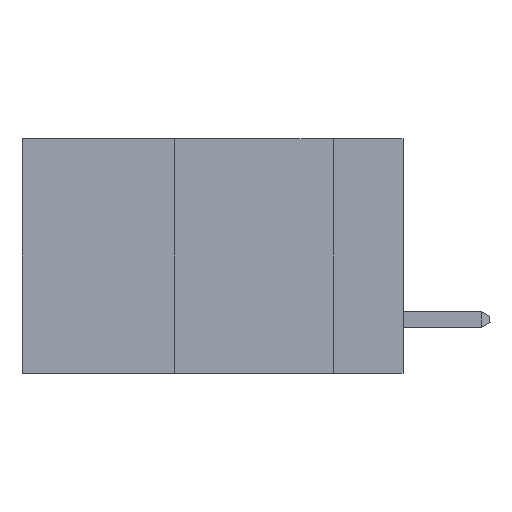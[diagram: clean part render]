
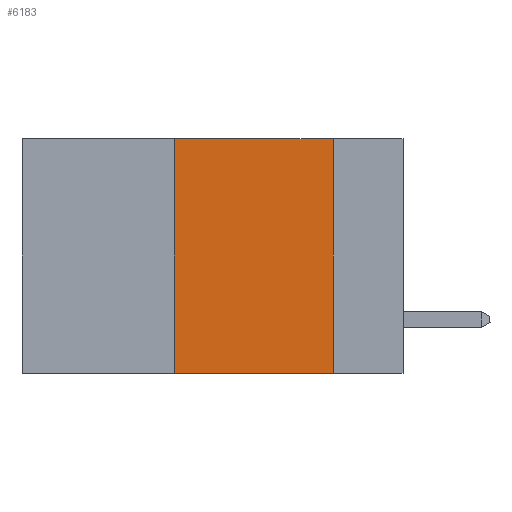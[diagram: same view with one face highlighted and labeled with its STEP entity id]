
A CAD part, left-side view. The second image highlights one B-rep face of the part: STEP entity #6183.
In plain terms, the highlighted planar face has unit normal (-1, 0, 0).
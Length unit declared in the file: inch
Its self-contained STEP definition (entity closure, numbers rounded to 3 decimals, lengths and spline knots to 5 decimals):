
#809 = VERTEX_POINT ( 'NONE', #3014 ) ;
#1024 = DIRECTION ( 'NONE',  ( 0., 0., 1. ) ) ;
#1670 = EDGE_CURVE ( 'NONE', #8490, #809, #32223, .T. ) ;
#1982 = VERTEX_POINT ( 'NONE', #28774 ) ;
#3014 = CARTESIAN_POINT ( 'NONE',  ( 0., 0.11, -0.37 ) ) ;
#3178 = CARTESIAN_POINT ( 'NONE',  ( 0., 0.6, -0.37 ) ) ;
#3404 = ORIENTED_EDGE ( 'NONE', *, *, #23162, .F. ) ;
#4191 = LINE ( 'NONE', #17182, #15447 ) ;
#5516 = VECTOR ( 'NONE', #15602, 39.37008 ) ;
#6183 = ADVANCED_FACE ( 'NONE', ( #23307 ), #29861, .F. ) ;
#6201 = CARTESIAN_POINT ( 'NONE',  ( 0., 0.11, 0. ) ) ;
#6342 = LINE ( 'NONE', #12565, #5516 ) ;
#6472 = EDGE_LOOP ( 'NONE', ( #3404, #15313, #8840, #18568 ) ) ;
#6728 = EDGE_CURVE ( 'NONE', #8490, #1982, #19120, .T. ) ;
#8490 = VERTEX_POINT ( 'NONE', #22607 ) ;
#8840 = ORIENTED_EDGE ( 'NONE', *, *, #6728, .F. ) ;
#9586 = DIRECTION ( 'NONE',  ( 0., 0., -1. ) ) ;
#12565 = CARTESIAN_POINT ( 'NONE',  ( 0., 0.11, 0. ) ) ;
#13324 = VECTOR ( 'NONE', #1024, 39.37008 ) ;
#14205 = EDGE_CURVE ( 'NONE', #1982, #18963, #4191, .T. ) ;
#14749 = DIRECTION ( 'NONE',  ( 1., 0., 0. ) ) ;
#15313 = ORIENTED_EDGE ( 'NONE', *, *, #14205, .F. ) ;
#15447 = VECTOR ( 'NONE', #22623, 39.37008 ) ;
#15602 = DIRECTION ( 'NONE',  ( 0., 0., -1. ) ) ;
#16715 = CARTESIAN_POINT ( 'NONE',  ( 0., 0.6, 0. ) ) ;
#17182 = CARTESIAN_POINT ( 'NONE',  ( 0., 0.6, 0. ) ) ;
#18568 = ORIENTED_EDGE ( 'NONE', *, *, #1670, .T. ) ;
#18963 = VERTEX_POINT ( 'NONE', #6201 ) ;
#19120 = LINE ( 'NONE', #24731, #13324 ) ;
#20783 = AXIS2_PLACEMENT_3D ( 'NONE', #16715, #14749, #9586 ) ;
#22607 = CARTESIAN_POINT ( 'NONE',  ( 0., 0.36, -0.37 ) ) ;
#22623 = DIRECTION ( 'NONE',  ( 0., -1., 0. ) ) ;
#23162 = EDGE_CURVE ( 'NONE', #18963, #809, #6342, .T. ) ;
#23307 = FACE_OUTER_BOUND ( 'NONE', #6472, .T. ) ;
#24481 = DIRECTION ( 'NONE',  ( 0., -1., 0. ) ) ;
#24731 = CARTESIAN_POINT ( 'NONE',  ( 0., 0.36, 0. ) ) ;
#24802 = VECTOR ( 'NONE', #24481, 39.37008 ) ;
#28774 = CARTESIAN_POINT ( 'NONE',  ( 0., 0.36, 0. ) ) ;
#29861 = PLANE ( 'NONE',  #20783 ) ;
#32223 = LINE ( 'NONE', #3178, #24802 ) ;
